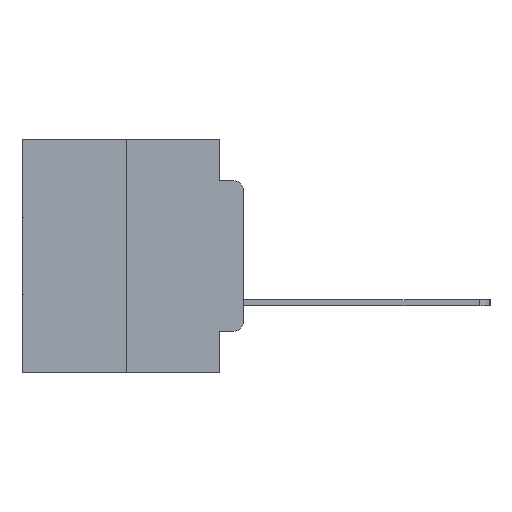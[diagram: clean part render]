
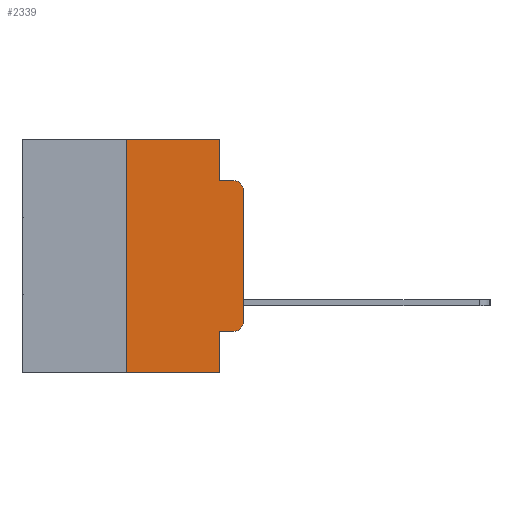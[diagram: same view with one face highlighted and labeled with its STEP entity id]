
A CAD part, left-side view. The second image highlights one B-rep face of the part: STEP entity #2339.
In plain terms, the highlighted planar face has unit normal (-1, 0, 0).
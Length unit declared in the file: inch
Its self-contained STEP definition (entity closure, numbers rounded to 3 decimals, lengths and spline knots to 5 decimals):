
#209 = DIRECTION ( 'NONE',  ( 0., 0., 1. ) ) ;
#277 = ORIENTED_EDGE ( 'NONE', *, *, #23386, .F. ) ;
#503 = CARTESIAN_POINT ( 'NONE',  ( 0., 0.473, 0. ) ) ;
#573 = CARTESIAN_POINT ( 'NONE',  ( 0., 0.051, -0.4115 ) ) ;
#997 = EDGE_CURVE ( 'NONE', #18933, #19931, #26204, .T. ) ;
#2339 = ADVANCED_FACE ( 'NONE', ( #3936 ), #7034, .F. ) ;
#2487 = EDGE_CURVE ( 'NONE', #9265, #19931, #17124, .T. ) ;
#2524 = CARTESIAN_POINT ( 'NONE',  ( 0., 0.473, -0.5 ) ) ;
#2830 = CARTESIAN_POINT ( 'NONE',  ( 0., 0., -0.1085 ) ) ;
#2898 = ORIENTED_EDGE ( 'NONE', *, *, #7020, .T. ) ;
#2950 = VECTOR ( 'NONE', #24988, 39.37008 ) ;
#3278 = CIRCLE ( 'NONE', #17407, 0.02 ) ;
#3661 = DIRECTION ( 'NONE',  ( 0., 0., -1. ) ) ;
#3936 = FACE_OUTER_BOUND ( 'NONE', #24449, .T. ) ;
#4282 = ORIENTED_EDGE ( 'NONE', *, *, #23739, .T. ) ;
#4650 = DIRECTION ( 'NONE',  ( -1., 0., 0. ) ) ;
#4683 = CARTESIAN_POINT ( 'NONE',  ( 0., 0.02, -0.1085 ) ) ;
#4750 = VERTEX_POINT ( 'NONE', #25336 ) ;
#4878 = CARTESIAN_POINT ( 'NONE',  ( 0., 0.051, 0. ) ) ;
#5427 = ORIENTED_EDGE ( 'NONE', *, *, #27599, .F. ) ;
#6255 = DIRECTION ( 'NONE',  ( 0., 0., -1. ) ) ;
#6852 = VERTEX_POINT ( 'NONE', #573 ) ;
#7020 = EDGE_CURVE ( 'NONE', #14326, #9265, #15228, .T. ) ;
#7034 = PLANE ( 'NONE',  #16229 ) ;
#7088 = DIRECTION ( 'NONE',  ( 0., 0., -1. ) ) ;
#7519 = DIRECTION ( 'NONE',  ( 0., 0., -1. ) ) ;
#7868 = CARTESIAN_POINT ( 'NONE',  ( 0., 0., 0. ) ) ;
#9023 = CARTESIAN_POINT ( 'NONE',  ( 0., 0.02, -0.3915 ) ) ;
#9265 = VERTEX_POINT ( 'NONE', #2830 ) ;
#9395 = LINE ( 'NONE', #21599, #14430 ) ;
#10115 = DIRECTION ( 'NONE',  ( 0., -1., 0. ) ) ;
#10275 = LINE ( 'NONE', #4878, #21035 ) ;
#10366 = ORIENTED_EDGE ( 'NONE', *, *, #21957, .F. ) ;
#11144 = DIRECTION ( 'NONE',  ( 0., 0., -1. ) ) ;
#11265 = DIRECTION ( 'NONE',  ( 0., -1., 0. ) ) ;
#11493 = CARTESIAN_POINT ( 'NONE',  ( 0., 0.02, -0.0885 ) ) ;
#12175 = ORIENTED_EDGE ( 'NONE', *, *, #2487, .T. ) ;
#12490 = CARTESIAN_POINT ( 'NONE',  ( 0., 0.051, -0.0885 ) ) ;
#13686 = DIRECTION ( 'NONE',  ( 0., -1., 0. ) ) ;
#14117 = VERTEX_POINT ( 'NONE', #16065 ) ;
#14326 = VERTEX_POINT ( 'NONE', #27302 ) ;
#14430 = VECTOR ( 'NONE', #23736, 39.37008 ) ;
#14436 = CARTESIAN_POINT ( 'NONE',  ( 0., 0.051, -0.0885 ) ) ;
#15228 = LINE ( 'NONE', #7868, #2950 ) ;
#15991 = DIRECTION ( 'NONE',  ( 1., 0., 0. ) ) ;
#16014 = CARTESIAN_POINT ( 'NONE',  ( 0., 0.473, 0. ) ) ;
#16065 = CARTESIAN_POINT ( 'NONE',  ( 0., 0.02, -0.4115 ) ) ;
#16229 = AXIS2_PLACEMENT_3D ( 'NONE', #16014, #15991, #7519 ) ;
#17124 = CIRCLE ( 'NONE', #27595, 0.02 ) ;
#17407 = AXIS2_PLACEMENT_3D ( 'NONE', #9023, #24002, #11144 ) ;
#17637 = EDGE_CURVE ( 'NONE', #14117, #14326, #3278, .T. ) ;
#18024 = VERTEX_POINT ( 'NONE', #28005 ) ;
#18933 = VERTEX_POINT ( 'NONE', #12490 ) ;
#19080 = EDGE_CURVE ( 'NONE', #6852, #14117, #9395, .T. ) ;
#19269 = EDGE_CURVE ( 'NONE', #18024, #21446, #26091, .T. ) ;
#19417 = ORIENTED_EDGE ( 'NONE', *, *, #19269, .F. ) ;
#19892 = VECTOR ( 'NONE', #10115, 39.37008 ) ;
#19931 = VERTEX_POINT ( 'NONE', #11493 ) ;
#20451 = VECTOR ( 'NONE', #13686, 39.37008 ) ;
#20987 = LINE ( 'NONE', #27570, #25931 ) ;
#21035 = VECTOR ( 'NONE', #7088, 39.37008 ) ;
#21113 = LINE ( 'NONE', #2524, #26054 ) ;
#21446 = VERTEX_POINT ( 'NONE', #21795 ) ;
#21599 = CARTESIAN_POINT ( 'NONE',  ( 0., 0.051, -0.4115 ) ) ;
#21795 = CARTESIAN_POINT ( 'NONE',  ( 0., 0.051, 0. ) ) ;
#21880 = CARTESIAN_POINT ( 'NONE',  ( 0., 0.25, 0. ) ) ;
#21957 = EDGE_CURVE ( 'NONE', #6852, #22500, #20987, .T. ) ;
#22500 = VERTEX_POINT ( 'NONE', #23155 ) ;
#23155 = CARTESIAN_POINT ( 'NONE',  ( 0., 0.051, -0.5 ) ) ;
#23386 = EDGE_CURVE ( 'NONE', #4750, #18024, #26549, .T. ) ;
#23736 = DIRECTION ( 'NONE',  ( 0., -1., 0. ) ) ;
#23739 = EDGE_CURVE ( 'NONE', #4750, #22500, #21113, .T. ) ;
#24002 = DIRECTION ( 'NONE',  ( -1., 0., 0. ) ) ;
#24415 = ORIENTED_EDGE ( 'NONE', *, *, #19080, .T. ) ;
#24449 = EDGE_LOOP ( 'NONE', ( #2898, #12175, #26214, #5427, #19417, #277, #4282, #10366, #24415, #28003 ) ) ;
#24988 = DIRECTION ( 'NONE',  ( 0., 0., 1. ) ) ;
#25336 = CARTESIAN_POINT ( 'NONE',  ( 0., 0.25, -0.5 ) ) ;
#25888 = VECTOR ( 'NONE', #209, 39.37008 ) ;
#25931 = VECTOR ( 'NONE', #6255, 39.37008 ) ;
#26054 = VECTOR ( 'NONE', #11265, 39.37008 ) ;
#26091 = LINE ( 'NONE', #503, #20451 ) ;
#26204 = LINE ( 'NONE', #14436, #19892 ) ;
#26214 = ORIENTED_EDGE ( 'NONE', *, *, #997, .F. ) ;
#26549 = LINE ( 'NONE', #21880, #25888 ) ;
#27302 = CARTESIAN_POINT ( 'NONE',  ( 0., 0., -0.3915 ) ) ;
#27570 = CARTESIAN_POINT ( 'NONE',  ( 0., 0.051, 0. ) ) ;
#27595 = AXIS2_PLACEMENT_3D ( 'NONE', #4683, #4650, #3661 ) ;
#27599 = EDGE_CURVE ( 'NONE', #21446, #18933, #10275, .T. ) ;
#28003 = ORIENTED_EDGE ( 'NONE', *, *, #17637, .T. ) ;
#28005 = CARTESIAN_POINT ( 'NONE',  ( 0., 0.25, 0. ) ) ;
